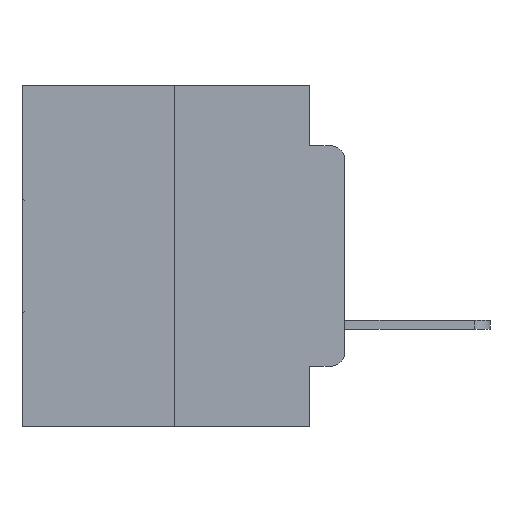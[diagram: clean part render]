
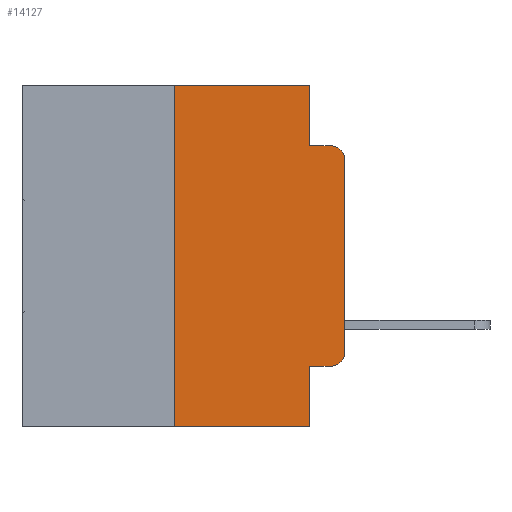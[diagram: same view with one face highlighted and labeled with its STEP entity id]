
A CAD part, left-side view. The second image highlights one B-rep face of the part: STEP entity #14127.
In plain terms, the highlighted planar face has unit normal (-1, 0, 0).
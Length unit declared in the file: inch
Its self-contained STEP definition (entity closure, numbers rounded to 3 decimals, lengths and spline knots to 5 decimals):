
#452 = CARTESIAN_POINT ( 'NONE',  ( 0., 0.051, 0. ) ) ;
#723 = VERTEX_POINT ( 'NONE', #17988 ) ;
#738 = AXIS2_PLACEMENT_3D ( 'NONE', #11918, #27240, #14148 ) ;
#1240 = CARTESIAN_POINT ( 'NONE',  ( 0., 0.051, 0. ) ) ;
#1419 = CARTESIAN_POINT ( 'NONE',  ( 0., 0.02, -0.3915 ) ) ;
#2699 = EDGE_CURVE ( 'NONE', #26499, #723, #7192, .T. ) ;
#3068 = EDGE_CURVE ( 'NONE', #20879, #12614, #27544, .T. ) ;
#3305 = ORIENTED_EDGE ( 'NONE', *, *, #24319, .T. ) ;
#3586 = VERTEX_POINT ( 'NONE', #452 ) ;
#3801 = DIRECTION ( 'NONE',  ( 0., 0., -1. ) ) ;
#3875 = VECTOR ( 'NONE', #7000, 39.37008 ) ;
#4426 = CARTESIAN_POINT ( 'NONE',  ( 0., 0.473, 0. ) ) ;
#5888 = LINE ( 'NONE', #8907, #22234 ) ;
#5987 = DIRECTION ( 'NONE',  ( 0., 0., -1. ) ) ;
#6028 = DIRECTION ( 'NONE',  ( 0., -1., 0. ) ) ;
#6870 = EDGE_CURVE ( 'NONE', #13068, #8476, #12629, .T. ) ;
#7000 = DIRECTION ( 'NONE',  ( 0., 0., -1. ) ) ;
#7067 = CARTESIAN_POINT ( 'NONE',  ( 0., 0.051, -0.0885 ) ) ;
#7192 = LINE ( 'NONE', #17236, #24903 ) ;
#7266 = EDGE_CURVE ( 'NONE', #20809, #20426, #25669, .T. ) ;
#7692 = CARTESIAN_POINT ( 'NONE',  ( 0., 0., -0.1085 ) ) ;
#7825 = EDGE_CURVE ( 'NONE', #723, #3586, #5888, .T. ) ;
#8015 = VECTOR ( 'NONE', #20399, 39.37008 ) ;
#8277 = LINE ( 'NONE', #1240, #19377 ) ;
#8476 = VERTEX_POINT ( 'NONE', #14116 ) ;
#8907 = CARTESIAN_POINT ( 'NONE',  ( 0., 0.473, 0. ) ) ;
#8958 = DIRECTION ( 'NONE',  ( 1., 0., 0. ) ) ;
#9326 = CIRCLE ( 'NONE', #738, 0.02 ) ;
#10632 = LINE ( 'NONE', #18094, #3875 ) ;
#10688 = VECTOR ( 'NONE', #13371, 39.37008 ) ;
#11154 = ORIENTED_EDGE ( 'NONE', *, *, #20324, .T. ) ;
#11918 = CARTESIAN_POINT ( 'NONE',  ( 0., 0.02, -0.1085 ) ) ;
#12510 = VECTOR ( 'NONE', #6028, 39.37008 ) ;
#12614 = VERTEX_POINT ( 'NONE', #7692 ) ;
#12629 = LINE ( 'NONE', #21194, #24363 ) ;
#13068 = VERTEX_POINT ( 'NONE', #7067 ) ;
#13235 = ORIENTED_EDGE ( 'NONE', *, *, #2699, .F. ) ;
#13269 = CARTESIAN_POINT ( 'NONE',  ( 0., 0.051, -0.4115 ) ) ;
#13371 = DIRECTION ( 'NONE',  ( 0., 0., 1. ) ) ;
#13576 = ORIENTED_EDGE ( 'NONE', *, *, #6870, .F. ) ;
#14116 = CARTESIAN_POINT ( 'NONE',  ( 0., 0.02, -0.0885 ) ) ;
#14127 = ADVANCED_FACE ( 'NONE', ( #15408 ), #28652, .F. ) ;
#14148 = DIRECTION ( 'NONE',  ( 0., 0., -1. ) ) ;
#14461 = AXIS2_PLACEMENT_3D ( 'NONE', #4426, #8958, #24509 ) ;
#15408 = FACE_OUTER_BOUND ( 'NONE', #24705, .T. ) ;
#15807 = CIRCLE ( 'NONE', #16607, 0.02 ) ;
#15850 = EDGE_CURVE ( 'NONE', #12614, #8476, #9326, .T. ) ;
#15963 = ORIENTED_EDGE ( 'NONE', *, *, #3068, .T. ) ;
#15988 = CARTESIAN_POINT ( 'NONE',  ( 0., 0.051, -0.4115 ) ) ;
#16108 = EDGE_CURVE ( 'NONE', #3586, #13068, #8277, .T. ) ;
#16492 = CARTESIAN_POINT ( 'NONE',  ( 0., 0.25, -0.5 ) ) ;
#16607 = AXIS2_PLACEMENT_3D ( 'NONE', #1419, #17256, #3801 ) ;
#17127 = CARTESIAN_POINT ( 'NONE',  ( 0., 0.473, -0.5 ) ) ;
#17236 = CARTESIAN_POINT ( 'NONE',  ( 0., 0.25, 0. ) ) ;
#17256 = DIRECTION ( 'NONE',  ( -1., 0., 0. ) ) ;
#17708 = ORIENTED_EDGE ( 'NONE', *, *, #7825, .F. ) ;
#17988 = CARTESIAN_POINT ( 'NONE',  ( 0., 0.25, 0. ) ) ;
#18050 = ORIENTED_EDGE ( 'NONE', *, *, #7266, .T. ) ;
#18094 = CARTESIAN_POINT ( 'NONE',  ( 0., 0.051, 0. ) ) ;
#18721 = ORIENTED_EDGE ( 'NONE', *, *, #15850, .T. ) ;
#18793 = CARTESIAN_POINT ( 'NONE',  ( 0., 0.051, -0.5 ) ) ;
#19042 = LINE ( 'NONE', #17127, #12510 ) ;
#19096 = DIRECTION ( 'NONE',  ( 0., 0., 1. ) ) ;
#19377 = VECTOR ( 'NONE', #5987, 39.37008 ) ;
#20157 = CARTESIAN_POINT ( 'NONE',  ( 0., 0., -0.3915 ) ) ;
#20324 = EDGE_CURVE ( 'NONE', #20426, #20879, #15807, .T. ) ;
#20399 = DIRECTION ( 'NONE',  ( 0., -1., 0. ) ) ;
#20426 = VERTEX_POINT ( 'NONE', #26349 ) ;
#20809 = VERTEX_POINT ( 'NONE', #13269 ) ;
#20879 = VERTEX_POINT ( 'NONE', #20157 ) ;
#21194 = CARTESIAN_POINT ( 'NONE',  ( 0., 0.051, -0.0885 ) ) ;
#21300 = CARTESIAN_POINT ( 'NONE',  ( 0., 0., 0. ) ) ;
#21626 = VERTEX_POINT ( 'NONE', #18793 ) ;
#22234 = VECTOR ( 'NONE', #22333, 39.37008 ) ;
#22333 = DIRECTION ( 'NONE',  ( 0., -1., 0. ) ) ;
#22581 = ORIENTED_EDGE ( 'NONE', *, *, #25844, .F. ) ;
#24319 = EDGE_CURVE ( 'NONE', #26499, #21626, #19042, .T. ) ;
#24363 = VECTOR ( 'NONE', #27670, 39.37008 ) ;
#24509 = DIRECTION ( 'NONE',  ( 0., 0., -1. ) ) ;
#24705 = EDGE_LOOP ( 'NONE', ( #15963, #18721, #13576, #26607, #17708, #13235, #3305, #22581, #18050, #11154 ) ) ;
#24903 = VECTOR ( 'NONE', #19096, 39.37008 ) ;
#25669 = LINE ( 'NONE', #15988, #8015 ) ;
#25844 = EDGE_CURVE ( 'NONE', #20809, #21626, #10632, .T. ) ;
#26349 = CARTESIAN_POINT ( 'NONE',  ( 0., 0.02, -0.4115 ) ) ;
#26499 = VERTEX_POINT ( 'NONE', #16492 ) ;
#26607 = ORIENTED_EDGE ( 'NONE', *, *, #16108, .F. ) ;
#27240 = DIRECTION ( 'NONE',  ( -1., 0., 0. ) ) ;
#27544 = LINE ( 'NONE', #21300, #10688 ) ;
#27670 = DIRECTION ( 'NONE',  ( 0., -1., 0. ) ) ;
#28652 = PLANE ( 'NONE',  #14461 ) ;
